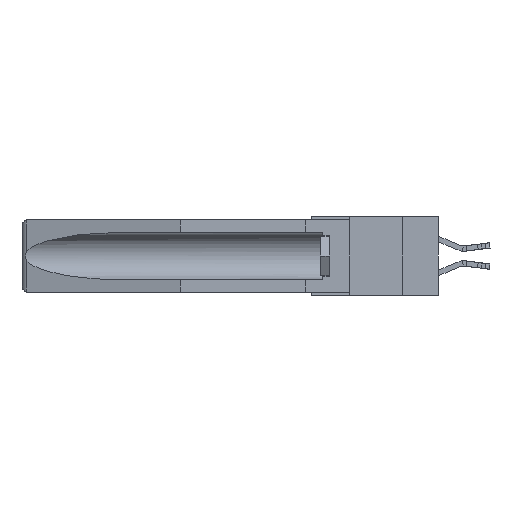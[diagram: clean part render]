
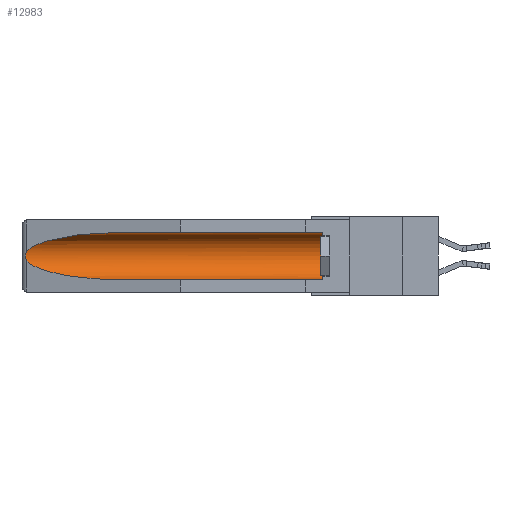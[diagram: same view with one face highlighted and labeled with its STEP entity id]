
A CAD part, left-side view. The second image highlights one B-rep face of the part: STEP entity #12983.
In plain terms, the highlighted cylindrical face has radius 2.857 mm (diameter 5.715 mm), a partial arc.
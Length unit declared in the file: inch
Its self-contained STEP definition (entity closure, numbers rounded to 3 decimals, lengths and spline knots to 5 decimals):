
#131 = AXIS2_PLACEMENT_3D ( 'NONE', #5929, #21378, #26256 ) ;
#1367 = EDGE_CURVE ( 'NONE', #25078, #27364, #15048, .T. ) ;
#1823 = CARTESIAN_POINT ( 'NONE',  ( 0.25451, 1.48313, -0.09465 ) ) ;
#2044 = ORIENTED_EDGE ( 'NONE', *, *, #31195, .T. ) ;
#2149 = EDGE_CURVE ( 'NONE', #9699, #11417, #4820, .T. ) ;
#2960 = CARTESIAN_POINT ( 'NONE',  ( 0.155, -0.30754, -0.059 ) ) ;
#3332 = VECTOR ( 'NONE', #6519, 39.37008 ) ;
#4216 = CARTESIAN_POINT ( 'NONE',  ( 0.155, 1.07973, -0.284 ) ) ;
#4820 =( BOUNDED_CURVE ( )  B_SPLINE_CURVE ( 3, ( #22475, #9389, #1823, #24693 ),
 .UNSPECIFIED., .F., .T. ) 
 B_SPLINE_CURVE_WITH_KNOTS ( ( 4, 4 ),
 ( 4.71239, 6.08839 ),
 .UNSPECIFIED. ) 
 CURVE ( )  GEOMETRIC_REPRESENTATION_ITEM ( )  RATIONAL_B_SPLINE_CURVE ( ( 1., 0.848, 0.848, 1. ) ) 
 REPRESENTATION_ITEM ( '' )  );
#5115 = CARTESIAN_POINT ( 'NONE',  ( 0.155, 0.126, -0.059 ) ) ;
#5929 = CARTESIAN_POINT ( 'NONE',  ( 0.155, 0.126, -0.1715 ) ) ;
#6272 = CARTESIAN_POINT ( 'NONE',  ( 0.155, 0.126, -0.284 ) ) ;
#6519 = DIRECTION ( 'NONE',  ( 0., 1., 0. ) ) ;
#7874 = DIRECTION ( 'NONE',  ( 0., 1., 0. ) ) ;
#8459 = CARTESIAN_POINT ( 'NONE',  ( 0.25451, 1.48313, -0.24835 ) ) ;
#8820 = CARTESIAN_POINT ( 'NONE',  ( 0.2675, 1.53308, -0.16763 ) ) ;
#9389 = CARTESIAN_POINT ( 'NONE',  ( 0.21114, 1.30732, -0.059 ) ) ;
#9699 = VERTEX_POINT ( 'NONE', #20658 ) ;
#9823 = ORIENTED_EDGE ( 'NONE', *, *, #14846, .T. ) ;
#9929 = VECTOR ( 'NONE', #7874, 39.37008 ) ;
#10025 = CIRCLE ( 'NONE', #131, 0.1125 ) ;
#11411 = CARTESIAN_POINT ( 'NONE',  ( 0.2673, 1.53269, -0.17917 ) ) ;
#11417 = VERTEX_POINT ( 'NONE', #29057 ) ;
#11780 = ORIENTED_EDGE ( 'NONE', *, *, #32415, .F. ) ;
#12983 = ADVANCED_FACE ( 'NONE', ( #25705 ), #26144, .F. ) ;
#13988 = VERTEX_POINT ( 'NONE', #6272 ) ;
#14709 = LINE ( 'NONE', #19113, #3332 ) ;
#14811 = CARTESIAN_POINT ( 'NONE',  ( 0.155, -0.30754, -0.1715 ) ) ;
#14846 = EDGE_CURVE ( 'NONE', #13988, #29410, #10025, .T. ) ;
#15044 = EDGE_CURVE ( 'NONE', #11417, #25078, #23723, .T. ) ;
#15048 =( BOUNDED_CURVE ( )  B_SPLINE_CURVE ( 3, ( #23953, #8459, #26594, #31182 ),
 .UNSPECIFIED., .F., .F. ) 
 B_SPLINE_CURVE_WITH_KNOTS ( ( 4, 4 ),
 ( 0.1948, 1.5708 ),
 .UNSPECIFIED. ) 
 CURVE ( )  GEOMETRIC_REPRESENTATION_ITEM ( )  RATIONAL_B_SPLINE_CURVE ( ( 1., 0.848, 0.848, 1. ) ) 
 REPRESENTATION_ITEM ( '' )  );
#16500 = CARTESIAN_POINT ( 'NONE',  ( 0.26597, 1.52961, -0.15275 ) ) ;
#16620 = CARTESIAN_POINT ( 'NONE',  ( 0.26655, 1.53094, -0.18657 ) ) ;
#16823 = LINE ( 'NONE', #2960, #9929 ) ;
#17327 = AXIS2_PLACEMENT_3D ( 'NONE', #14811, #19700, #27635 ) ;
#17919 = CARTESIAN_POINT ( 'NONE',  ( 0.26537, 1.52718, -0.19328 ) ) ;
#19106 = CARTESIAN_POINT ( 'NONE',  ( 0.26654, 1.53092, -0.15636 ) ) ;
#19113 = CARTESIAN_POINT ( 'NONE',  ( 0.155, -0.30754, -0.284 ) ) ;
#19700 = DIRECTION ( 'NONE',  ( 0., 1., 0. ) ) ;
#20658 = CARTESIAN_POINT ( 'NONE',  ( 0.155, 1.07973, -0.059 ) ) ;
#21378 = DIRECTION ( 'NONE',  ( 0., -1., 0. ) ) ;
#22475 = CARTESIAN_POINT ( 'NONE',  ( 0.155, 1.07973, -0.059 ) ) ;
#22745 = ORIENTED_EDGE ( 'NONE', *, *, #15044, .T. ) ;
#23723 = B_SPLINE_CURVE_WITH_KNOTS ( 'NONE', 3,
 ( #24206, #16500, #19106, #24331, #8820, #26948, #11411, #16620, #32653, #30296 ),
 .UNSPECIFIED., .F., .F.,
 ( 4, 2, 2, 2, 4 ),
 ( 0., 0.00029, 0.00058, 0.00087, 0.00117 ),
 .UNSPECIFIED. ) ;
#23953 = CARTESIAN_POINT ( 'NONE',  ( 0.26537, 1.52718, -0.19328 ) ) ;
#24206 = CARTESIAN_POINT ( 'NONE',  ( 0.26537, 1.52718, -0.14972 ) ) ;
#24331 = CARTESIAN_POINT ( 'NONE',  ( 0.2673, 1.5327, -0.16383 ) ) ;
#24693 = CARTESIAN_POINT ( 'NONE',  ( 0.26537, 1.52718, -0.14972 ) ) ;
#25078 = VERTEX_POINT ( 'NONE', #17919 ) ;
#25705 = FACE_OUTER_BOUND ( 'NONE', #31241, .T. ) ;
#26144 = CYLINDRICAL_SURFACE ( 'NONE', #17327, 0.1125 ) ;
#26256 = DIRECTION ( 'NONE',  ( 0., 0., 1. ) ) ;
#26594 = CARTESIAN_POINT ( 'NONE',  ( 0.21114, 1.30732, -0.284 ) ) ;
#26948 = CARTESIAN_POINT ( 'NONE',  ( 0.2675, 1.53308, -0.17534 ) ) ;
#27364 = VERTEX_POINT ( 'NONE', #4216 ) ;
#27635 = DIRECTION ( 'NONE',  ( 0., 0., 1. ) ) ;
#27721 = ORIENTED_EDGE ( 'NONE', *, *, #1367, .T. ) ;
#29057 = CARTESIAN_POINT ( 'NONE',  ( 0.26537, 1.52718, -0.14972 ) ) ;
#29410 = VERTEX_POINT ( 'NONE', #5115 ) ;
#29572 = ORIENTED_EDGE ( 'NONE', *, *, #2149, .T. ) ;
#30296 = CARTESIAN_POINT ( 'NONE',  ( 0.26537, 1.52718, -0.19328 ) ) ;
#31182 = CARTESIAN_POINT ( 'NONE',  ( 0.155, 1.07973, -0.284 ) ) ;
#31195 = EDGE_CURVE ( 'NONE', #29410, #9699, #16823, .T. ) ;
#31241 = EDGE_LOOP ( 'NONE', ( #29572, #22745, #27721, #11780, #9823, #2044 ) ) ;
#32415 = EDGE_CURVE ( 'NONE', #13988, #27364, #14709, .T. ) ;
#32653 = CARTESIAN_POINT ( 'NONE',  ( 0.26597, 1.5296, -0.19026 ) ) ;
